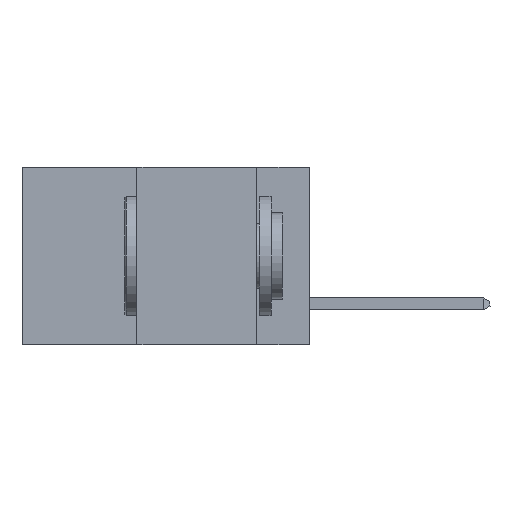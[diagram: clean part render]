
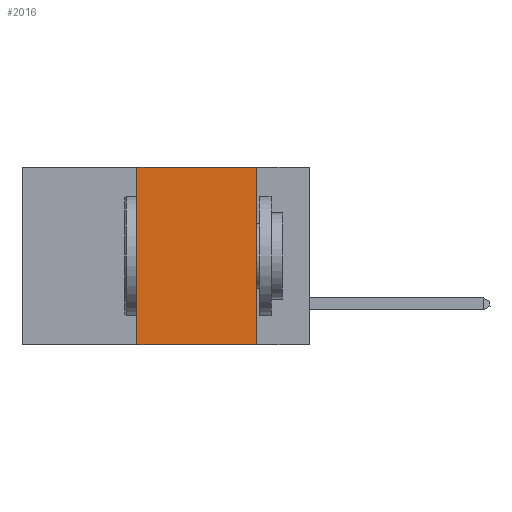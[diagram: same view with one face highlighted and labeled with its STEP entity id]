
A CAD part, left-side view. The second image highlights one B-rep face of the part: STEP entity #2016.
In plain terms, the highlighted planar face has unit normal (-1, 0, 0).
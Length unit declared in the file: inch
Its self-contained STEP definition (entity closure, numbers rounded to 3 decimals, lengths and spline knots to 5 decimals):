
#517 = FACE_OUTER_BOUND ( 'NONE', #4420, .T. ) ;
#1371 = CARTESIAN_POINT ( 'NONE',  ( 0., 0.11, 0. ) ) ;
#1500 = VERTEX_POINT ( 'NONE', #6125 ) ;
#2016 = ADVANCED_FACE ( 'NONE', ( #517 ), #6543, .F. ) ;
#3274 = DIRECTION ( 'NONE',  ( 0., -1., 0. ) ) ;
#3348 = ORIENTED_EDGE ( 'NONE', *, *, #4259, .T. ) ;
#4259 = EDGE_CURVE ( 'NONE', #5963, #1500, #36256, .T. ) ;
#4420 = EDGE_LOOP ( 'NONE', ( #28680, #28481, #30187, #3348 ) ) ;
#4423 = DIRECTION ( 'NONE',  ( 0., 0., -1. ) ) ;
#5685 = DIRECTION ( 'NONE',  ( 0., 0., -1. ) ) ;
#5963 = VERTEX_POINT ( 'NONE', #13784 ) ;
#6125 = CARTESIAN_POINT ( 'NONE',  ( 0., 0.11, -0.37 ) ) ;
#6138 = DIRECTION ( 'NONE',  ( 1., 0., 0. ) ) ;
#6167 = CARTESIAN_POINT ( 'NONE',  ( 0., 0.6, 0. ) ) ;
#6543 = PLANE ( 'NONE',  #20454 ) ;
#7097 = VECTOR ( 'NONE', #14136, 39.37008 ) ;
#9618 = LINE ( 'NONE', #21250, #25441 ) ;
#10005 = EDGE_CURVE ( 'NONE', #30618, #1500, #15415, .T. ) ;
#12674 = EDGE_CURVE ( 'NONE', #5963, #34984, #32232, .T. ) ;
#13784 = CARTESIAN_POINT ( 'NONE',  ( 0., 0.36, -0.37 ) ) ;
#13883 = CARTESIAN_POINT ( 'NONE',  ( 0., 0.36, 0. ) ) ;
#14136 = DIRECTION ( 'NONE',  ( 0., 0., 1. ) ) ;
#15415 = LINE ( 'NONE', #1371, #30345 ) ;
#17825 = DIRECTION ( 'NONE',  ( 0., -1., 0. ) ) ;
#18451 = CARTESIAN_POINT ( 'NONE',  ( 0., 0.11, 0. ) ) ;
#19569 = VECTOR ( 'NONE', #17825, 39.37008 ) ;
#20454 = AXIS2_PLACEMENT_3D ( 'NONE', #6167, #6138, #5685 ) ;
#21250 = CARTESIAN_POINT ( 'NONE',  ( 0., 0.6, 0. ) ) ;
#23828 = CARTESIAN_POINT ( 'NONE',  ( 0., 0.6, -0.37 ) ) ;
#25441 = VECTOR ( 'NONE', #3274, 39.37008 ) ;
#28481 = ORIENTED_EDGE ( 'NONE', *, *, #36440, .F. ) ;
#28680 = ORIENTED_EDGE ( 'NONE', *, *, #10005, .F. ) ;
#30187 = ORIENTED_EDGE ( 'NONE', *, *, #12674, .F. ) ;
#30345 = VECTOR ( 'NONE', #4423, 39.37008 ) ;
#30618 = VERTEX_POINT ( 'NONE', #18451 ) ;
#32232 = LINE ( 'NONE', #37842, #7097 ) ;
#34984 = VERTEX_POINT ( 'NONE', #13883 ) ;
#36256 = LINE ( 'NONE', #23828, #19569 ) ;
#36440 = EDGE_CURVE ( 'NONE', #34984, #30618, #9618, .T. ) ;
#37842 = CARTESIAN_POINT ( 'NONE',  ( 0., 0.36, 0. ) ) ;
